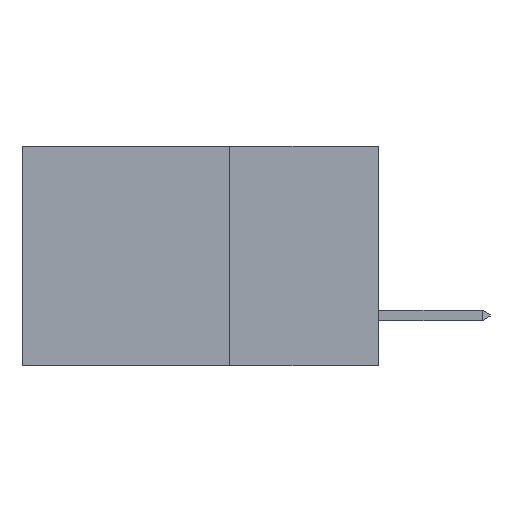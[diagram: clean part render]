
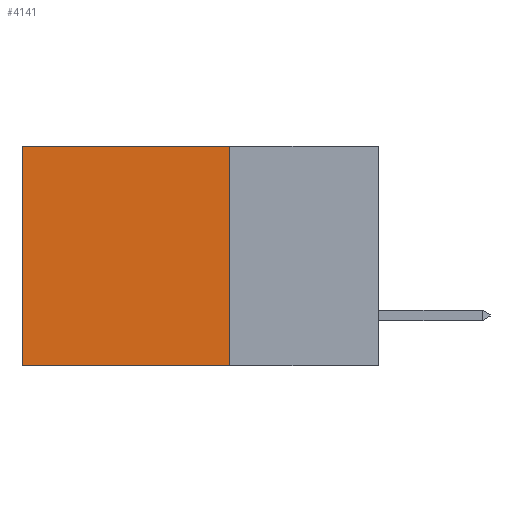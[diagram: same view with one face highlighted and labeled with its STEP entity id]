
A CAD part, left-side view. The second image highlights one B-rep face of the part: STEP entity #4141.
In plain terms, the highlighted planar face has unit normal (-1, 0, 0).
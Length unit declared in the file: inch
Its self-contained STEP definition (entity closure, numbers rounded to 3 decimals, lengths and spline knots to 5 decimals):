
#1023 = EDGE_CURVE ( 'NONE', #22986, #29991, #6171, .T. ) ;
#1453 = CARTESIAN_POINT ( 'NONE',  ( 0.298, 0.25, 0. ) ) ;
#2596 = CARTESIAN_POINT ( 'NONE',  ( 0.298, 0.25, 0. ) ) ;
#3660 = EDGE_CURVE ( 'NONE', #31539, #29991, #27227, .T. ) ;
#4141 = ADVANCED_FACE ( 'NONE', ( #29020 ), #15079, .F. ) ;
#6171 = LINE ( 'NONE', #13395, #17227 ) ;
#7855 = DIRECTION ( 'NONE',  ( 0., 0., -1. ) ) ;
#9242 = AXIS2_PLACEMENT_3D ( 'NONE', #1453, #15011, #17608 ) ;
#10198 = ORIENTED_EDGE ( 'NONE', *, *, #30626, .T. ) ;
#10559 = DIRECTION ( 'NONE',  ( 0., 0., -1. ) ) ;
#11114 = EDGE_CURVE ( 'NONE', #30568, #31539, #14037, .T. ) ;
#13395 = CARTESIAN_POINT ( 'NONE',  ( 0.298, 0.6, 0. ) ) ;
#14037 = LINE ( 'NONE', #22934, #21589 ) ;
#14470 = EDGE_LOOP ( 'NONE', ( #21546, #31120, #18787, #10198 ) ) ;
#14880 = CARTESIAN_POINT ( 'NONE',  ( 0.298, 0.25, 0. ) ) ;
#15011 = DIRECTION ( 'NONE',  ( 1., 0., 0. ) ) ;
#15079 = PLANE ( 'NONE',  #9242 ) ;
#15673 = DIRECTION ( 'NONE',  ( 0., 1., 0. ) ) ;
#17124 = VECTOR ( 'NONE', #22711, 39.37008 ) ;
#17227 = VECTOR ( 'NONE', #10559, 39.37008 ) ;
#17608 = DIRECTION ( 'NONE',  ( 0., 0., -1. ) ) ;
#17698 = CARTESIAN_POINT ( 'NONE',  ( 0.298, 0.6, -0.37 ) ) ;
#18787 = ORIENTED_EDGE ( 'NONE', *, *, #11114, .F. ) ;
#19204 = VECTOR ( 'NONE', #15673, 39.37008 ) ;
#19213 = CARTESIAN_POINT ( 'NONE',  ( 0.298, 0.25, -0.37 ) ) ;
#21546 = ORIENTED_EDGE ( 'NONE', *, *, #1023, .T. ) ;
#21589 = VECTOR ( 'NONE', #7855, 39.37008 ) ;
#22711 = DIRECTION ( 'NONE',  ( 0., 1., 0. ) ) ;
#22934 = CARTESIAN_POINT ( 'NONE',  ( 0.298, 0.25, 0. ) ) ;
#22986 = VERTEX_POINT ( 'NONE', #27986 ) ;
#25268 = LINE ( 'NONE', #2596, #17124 ) ;
#27227 = LINE ( 'NONE', #28645, #19204 ) ;
#27986 = CARTESIAN_POINT ( 'NONE',  ( 0.298, 0.6, 0. ) ) ;
#28645 = CARTESIAN_POINT ( 'NONE',  ( 0.298, 0.25, -0.37 ) ) ;
#29020 = FACE_OUTER_BOUND ( 'NONE', #14470, .T. ) ;
#29991 = VERTEX_POINT ( 'NONE', #17698 ) ;
#30568 = VERTEX_POINT ( 'NONE', #14880 ) ;
#30626 = EDGE_CURVE ( 'NONE', #30568, #22986, #25268, .T. ) ;
#31120 = ORIENTED_EDGE ( 'NONE', *, *, #3660, .F. ) ;
#31539 = VERTEX_POINT ( 'NONE', #19213 ) ;
